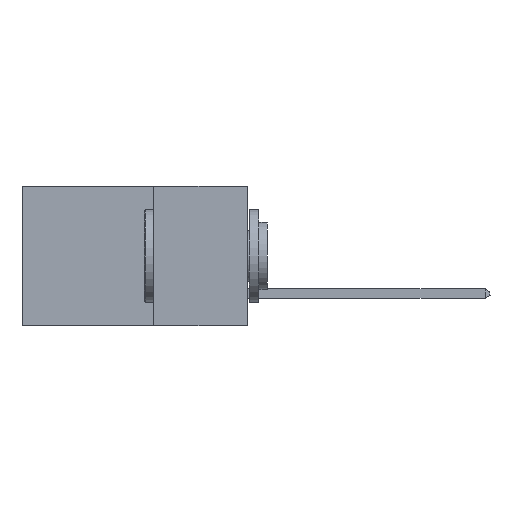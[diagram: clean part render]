
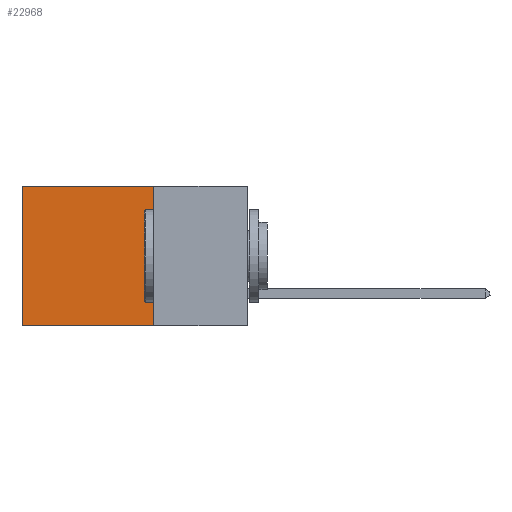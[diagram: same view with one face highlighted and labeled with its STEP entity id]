
A CAD part, left-side view. The second image highlights one B-rep face of the part: STEP entity #22968.
In plain terms, the highlighted planar face has unit normal (-1, 0, 0).
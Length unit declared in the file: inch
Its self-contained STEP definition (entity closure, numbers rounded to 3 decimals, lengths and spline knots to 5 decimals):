
#92 = EDGE_CURVE ( 'NONE', #8613, #730, #7182, .T. ) ;
#174 = ORIENTED_EDGE ( 'NONE', *, *, #92, .F. ) ;
#298 = VECTOR ( 'NONE', #904, 39.37008 ) ;
#633 = VECTOR ( 'NONE', #21154, 39.37008 ) ;
#647 = ORIENTED_EDGE ( 'NONE', *, *, #15405, .F. ) ;
#730 = VERTEX_POINT ( 'NONE', #10132 ) ;
#823 = CARTESIAN_POINT ( 'NONE',  ( 0.298, 0.25, 0. ) ) ;
#904 = DIRECTION ( 'NONE',  ( 0., 1., 0. ) ) ;
#2293 = ORIENTED_EDGE ( 'NONE', *, *, #14445, .T. ) ;
#2470 = ORIENTED_EDGE ( 'NONE', *, *, #8489, .T. ) ;
#2856 = CARTESIAN_POINT ( 'NONE',  ( 0.298, 0.6, 0. ) ) ;
#3106 = CARTESIAN_POINT ( 'NONE',  ( 0.298, 0.25, -0.37 ) ) ;
#3339 = CARTESIAN_POINT ( 'NONE',  ( 0.298, 0.25, 0. ) ) ;
#3766 = PLANE ( 'NONE',  #22414 ) ;
#3850 = CARTESIAN_POINT ( 'NONE',  ( 0.298, 0.25, 0. ) ) ;
#4212 = LINE ( 'NONE', #16716, #298 ) ;
#5243 = VECTOR ( 'NONE', #20997, 39.37008 ) ;
#5414 = LINE ( 'NONE', #2856, #633 ) ;
#7182 = LINE ( 'NONE', #3339, #5243 ) ;
#8483 = CARTESIAN_POINT ( 'NONE',  ( 0.298, 0.6, -0.37 ) ) ;
#8489 = EDGE_CURVE ( 'NONE', #8613, #23135, #4212, .T. ) ;
#8613 = VERTEX_POINT ( 'NONE', #823 ) ;
#10132 = CARTESIAN_POINT ( 'NONE',  ( 0.298, 0.25, -0.37 ) ) ;
#10899 = DIRECTION ( 'NONE',  ( 0., 0., -1. ) ) ;
#12426 = LINE ( 'NONE', #3106, #21181 ) ;
#14445 = EDGE_CURVE ( 'NONE', #23135, #19527, #5414, .T. ) ;
#15405 = EDGE_CURVE ( 'NONE', #730, #19527, #12426, .T. ) ;
#16427 = DIRECTION ( 'NONE',  ( 1., 0., 0. ) ) ;
#16716 = CARTESIAN_POINT ( 'NONE',  ( 0.298, 0.25, 0. ) ) ;
#16830 = FACE_OUTER_BOUND ( 'NONE', #21866, .T. ) ;
#19527 = VERTEX_POINT ( 'NONE', #8483 ) ;
#20892 = CARTESIAN_POINT ( 'NONE',  ( 0.298, 0.6, 0. ) ) ;
#20997 = DIRECTION ( 'NONE',  ( 0., 0., -1. ) ) ;
#21154 = DIRECTION ( 'NONE',  ( 0., 0., -1. ) ) ;
#21181 = VECTOR ( 'NONE', #22975, 39.37008 ) ;
#21866 = EDGE_LOOP ( 'NONE', ( #2293, #647, #174, #2470 ) ) ;
#22414 = AXIS2_PLACEMENT_3D ( 'NONE', #3850, #16427, #10899 ) ;
#22968 = ADVANCED_FACE ( 'NONE', ( #16830 ), #3766, .F. ) ;
#22975 = DIRECTION ( 'NONE',  ( 0., 1., 0. ) ) ;
#23135 = VERTEX_POINT ( 'NONE', #20892 ) ;
